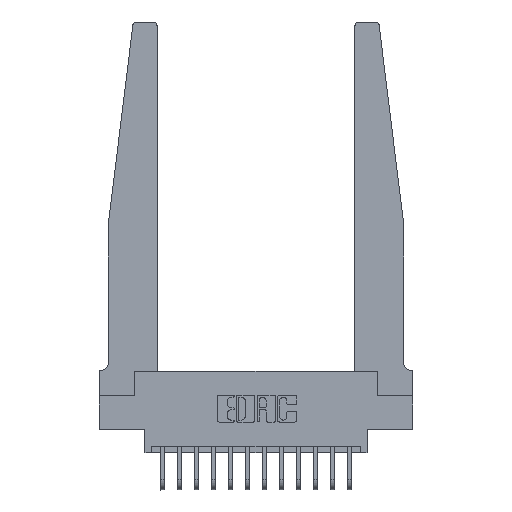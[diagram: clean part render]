
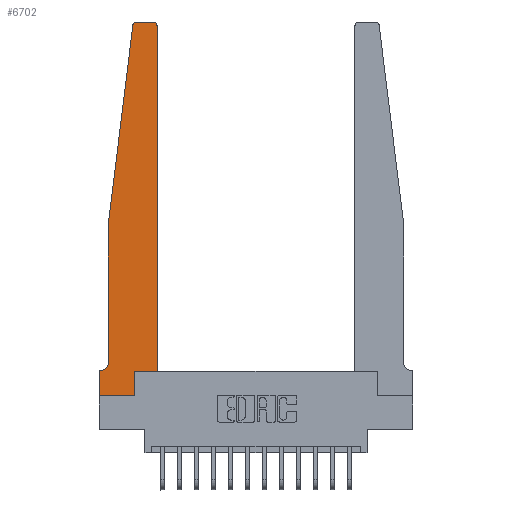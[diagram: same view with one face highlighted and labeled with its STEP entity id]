
A CAD part, top view. The second image highlights one B-rep face of the part: STEP entity #6702.
In plain terms, the highlighted planar face has unit normal (0, 0, 1).
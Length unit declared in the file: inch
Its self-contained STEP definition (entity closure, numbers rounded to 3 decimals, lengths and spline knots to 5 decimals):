
#280 = DIRECTION ( 'NONE',  ( 0., 0., 1. ) ) ;
#398 = AXIS2_PLACEMENT_3D ( 'NONE', #4300, #5938, #13648 ) ;
#603 = VERTEX_POINT ( 'NONE', #10738 ) ;
#903 = CARTESIAN_POINT ( 'NONE',  ( 0.065, 1.25, 0.37 ) ) ;
#989 = DIRECTION ( 'NONE',  ( 0., 0., 1. ) ) ;
#1044 = ORIENTED_EDGE ( 'NONE', *, *, #8062, .T. ) ;
#1139 = DIRECTION ( 'NONE',  ( 0., -1., 0. ) ) ;
#1317 = LINE ( 'NONE', #6361, #5073 ) ;
#1368 = VERTEX_POINT ( 'NONE', #12760 ) ;
#1371 = DIRECTION ( 'NONE',  ( 1., 0., 0. ) ) ;
#1386 = ORIENTED_EDGE ( 'NONE', *, *, #15175, .T. ) ;
#1462 = CARTESIAN_POINT ( 'NONE',  ( 0.25, 2.75, 0.37 ) ) ;
#1670 = VERTEX_POINT ( 'NONE', #11130 ) ;
#1686 = VECTOR ( 'NONE', #15505, 39.37008 ) ;
#1709 = ORIENTED_EDGE ( 'NONE', *, *, #5393, .T. ) ;
#2295 = EDGE_LOOP ( 'NONE', ( #4385, #1044, #1386, #11951, #5668, #1709, #12497, #16270, #10180, #5427, #3287, #5014 ) ) ;
#2514 = VECTOR ( 'NONE', #15736, 39.37008 ) ;
#2780 = VECTOR ( 'NONE', #6752, 39.37008 ) ;
#2813 = CARTESIAN_POINT ( 'NONE',  ( 0.2605, 0.18, 0.37 ) ) ;
#2824 = AXIS2_PLACEMENT_3D ( 'NONE', #11915, #280, #6591 ) ;
#2952 = CARTESIAN_POINT ( 'NONE',  ( 0.2605, 0., 0.37 ) ) ;
#2966 = EDGE_CURVE ( 'NONE', #1368, #3412, #13705, .T. ) ;
#3287 = ORIENTED_EDGE ( 'NONE', *, *, #10945, .T. ) ;
#3412 = VERTEX_POINT ( 'NONE', #13411 ) ;
#3525 = CARTESIAN_POINT ( 'NONE',  ( 0., 0.1875, 0.37 ) ) ;
#3641 = CIRCLE ( 'NONE', #2824, 0.03 ) ;
#3693 = LINE ( 'NONE', #7657, #1686 ) ;
#4300 = CARTESIAN_POINT ( 'NONE',  ( 0.015, 0.2375, 0.37 ) ) ;
#4385 = ORIENTED_EDGE ( 'NONE', *, *, #5815, .T. ) ;
#4401 = VECTOR ( 'NONE', #7994, 39.37008 ) ;
#4592 = LINE ( 'NONE', #7610, #6512 ) ;
#4669 = VERTEX_POINT ( 'NONE', #12641 ) ;
#4897 = DIRECTION ( 'NONE',  ( 0., 0., 1. ) ) ;
#4987 = DIRECTION ( 'NONE',  ( 0., 1., 0. ) ) ;
#5014 = ORIENTED_EDGE ( 'NONE', *, *, #2966, .T. ) ;
#5073 = VECTOR ( 'NONE', #4987, 39.37008 ) ;
#5202 = AXIS2_PLACEMENT_3D ( 'NONE', #11506, #989, #1371 ) ;
#5246 = EDGE_CURVE ( 'NONE', #7898, #11640, #3693, .T. ) ;
#5393 = EDGE_CURVE ( 'NONE', #1670, #603, #9539, .T. ) ;
#5427 = ORIENTED_EDGE ( 'NONE', *, *, #9432, .T. ) ;
#5528 = AXIS2_PLACEMENT_3D ( 'NONE', #3525, #4897, #9882 ) ;
#5668 = ORIENTED_EDGE ( 'NONE', *, *, #7704, .T. ) ;
#5815 = EDGE_CURVE ( 'NONE', #3412, #6005, #6827, .T. ) ;
#5880 = EDGE_CURVE ( 'NONE', #6100, #11102, #13355, .T. ) ;
#5938 = DIRECTION ( 'NONE',  ( 0., 0., -1. ) ) ;
#6005 = VERTEX_POINT ( 'NONE', #8825 ) ;
#6016 = EDGE_CURVE ( 'NONE', #4669, #6100, #10104, .T. ) ;
#6100 = VERTEX_POINT ( 'NONE', #2952 ) ;
#6361 = CARTESIAN_POINT ( 'NONE',  ( 0.425, 0.18, 0.37 ) ) ;
#6512 = VECTOR ( 'NONE', #8741, 39.37008 ) ;
#6518 = VERTEX_POINT ( 'NONE', #9115 ) ;
#6581 = CARTESIAN_POINT ( 'NONE',  ( 0.24675, 2.72367, 0.37 ) ) ;
#6591 = DIRECTION ( 'NONE',  ( 1., 0., 0. ) ) ;
#6700 = EDGE_CURVE ( 'NONE', #603, #4669, #12609, .T. ) ;
#6702 = ADVANCED_FACE ( 'NONE', ( #16532 ), #14136, .T. ) ;
#6752 = DIRECTION ( 'NONE',  ( -1., 0., 0. ) ) ;
#6827 = LINE ( 'NONE', #1462, #2780 ) ;
#7610 = CARTESIAN_POINT ( 'NONE',  ( 0.065, 1.25, 0.37 ) ) ;
#7657 = CARTESIAN_POINT ( 'NONE',  ( 0.065, 1.25, 0.37 ) ) ;
#7704 = EDGE_CURVE ( 'NONE', #11640, #1670, #14570, .T. ) ;
#7803 = VECTOR ( 'NONE', #8599, 39.37008 ) ;
#7898 = VERTEX_POINT ( 'NONE', #903 ) ;
#7994 = DIRECTION ( 'NONE',  ( -1., 0., 0. ) ) ;
#8062 = EDGE_CURVE ( 'NONE', #6005, #15080, #3641, .T. ) ;
#8561 = VECTOR ( 'NONE', #15301, 39.37008 ) ;
#8599 = DIRECTION ( 'NONE',  ( 1., 0., 0. ) ) ;
#8741 = DIRECTION ( 'NONE',  ( -0.122, -0.992, 0. ) ) ;
#8825 = CARTESIAN_POINT ( 'NONE',  ( 0.27653, 2.75, 0.37 ) ) ;
#9115 = CARTESIAN_POINT ( 'NONE',  ( 0.425, 0.18, 0.37 ) ) ;
#9432 = EDGE_CURVE ( 'NONE', #11102, #6518, #10984, .T. ) ;
#9539 = LINE ( 'NONE', #13114, #4401 ) ;
#9882 = DIRECTION ( 'NONE',  ( 1., 0., 0. ) ) ;
#10104 = LINE ( 'NONE', #10195, #8561 ) ;
#10142 = CARTESIAN_POINT ( 'NONE',  ( 0., 0., 0.37 ) ) ;
#10180 = ORIENTED_EDGE ( 'NONE', *, *, #5880, .T. ) ;
#10195 = CARTESIAN_POINT ( 'NONE',  ( 0., 0., 0.37 ) ) ;
#10738 = CARTESIAN_POINT ( 'NONE',  ( 0., 0.1875, 0.37 ) ) ;
#10945 = EDGE_CURVE ( 'NONE', #6518, #1368, #1317, .T. ) ;
#10984 = LINE ( 'NONE', #16178, #7803 ) ;
#11102 = VERTEX_POINT ( 'NONE', #12249 ) ;
#11130 = CARTESIAN_POINT ( 'NONE',  ( 0.015, 0.1875, 0.37 ) ) ;
#11506 = CARTESIAN_POINT ( 'NONE',  ( 0.395, 2.72, 0.37 ) ) ;
#11640 = VERTEX_POINT ( 'NONE', #16483 ) ;
#11915 = CARTESIAN_POINT ( 'NONE',  ( 0.27653, 2.72, 0.37 ) ) ;
#11951 = ORIENTED_EDGE ( 'NONE', *, *, #5246, .T. ) ;
#12249 = CARTESIAN_POINT ( 'NONE',  ( 0.2605, 0.18, 0.37 ) ) ;
#12497 = ORIENTED_EDGE ( 'NONE', *, *, #6700, .T. ) ;
#12609 = LINE ( 'NONE', #10142, #15373 ) ;
#12641 = CARTESIAN_POINT ( 'NONE',  ( 0., 0., 0.37 ) ) ;
#12760 = CARTESIAN_POINT ( 'NONE',  ( 0.425, 2.72, 0.37 ) ) ;
#13114 = CARTESIAN_POINT ( 'NONE',  ( 0.065, 0.1875, 0.37 ) ) ;
#13355 = LINE ( 'NONE', #2813, #2514 ) ;
#13411 = CARTESIAN_POINT ( 'NONE',  ( 0.395, 2.75, 0.37 ) ) ;
#13648 = DIRECTION ( 'NONE',  ( -1., 0., 0. ) ) ;
#13705 = CIRCLE ( 'NONE', #5202, 0.03 ) ;
#14136 = PLANE ( 'NONE',  #5528 ) ;
#14570 = CIRCLE ( 'NONE', #398, 0.05 ) ;
#15080 = VERTEX_POINT ( 'NONE', #6581 ) ;
#15175 = EDGE_CURVE ( 'NONE', #15080, #7898, #4592, .T. ) ;
#15301 = DIRECTION ( 'NONE',  ( 1., 0., 0. ) ) ;
#15373 = VECTOR ( 'NONE', #1139, 39.37008 ) ;
#15505 = DIRECTION ( 'NONE',  ( 0., -1., 0. ) ) ;
#15736 = DIRECTION ( 'NONE',  ( 0., 1., 0. ) ) ;
#16178 = CARTESIAN_POINT ( 'NONE',  ( 0.425, 0.18, 0.37 ) ) ;
#16270 = ORIENTED_EDGE ( 'NONE', *, *, #6016, .T. ) ;
#16483 = CARTESIAN_POINT ( 'NONE',  ( 0.065, 0.2375, 0.37 ) ) ;
#16532 = FACE_OUTER_BOUND ( 'NONE', #2295, .T. ) ;
